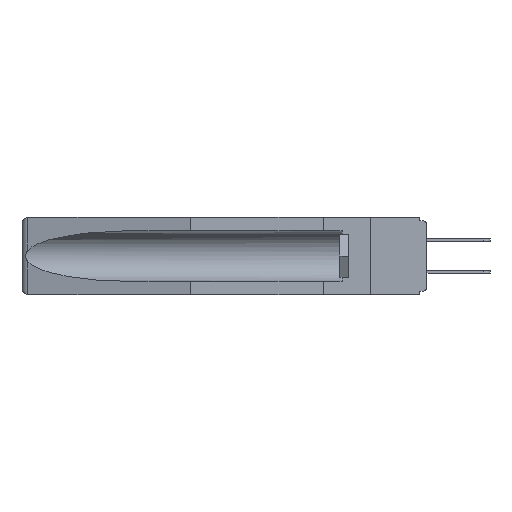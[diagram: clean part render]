
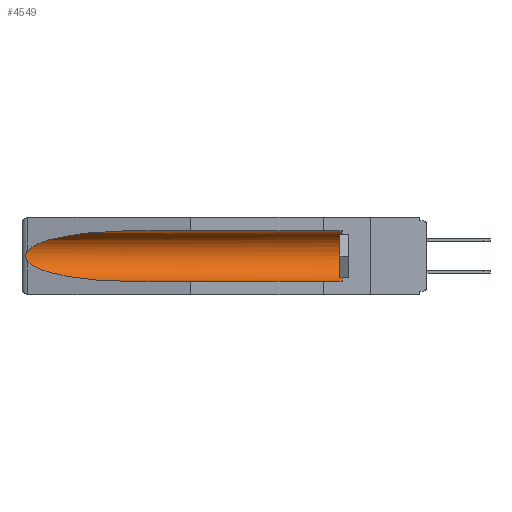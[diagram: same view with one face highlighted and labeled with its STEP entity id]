
A CAD part, left-side view. The second image highlights one B-rep face of the part: STEP entity #4549.
In plain terms, the highlighted cylindrical face has radius 2.857 mm (diameter 5.715 mm), a partial arc.
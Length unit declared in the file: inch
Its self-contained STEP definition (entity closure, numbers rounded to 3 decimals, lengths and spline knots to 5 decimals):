
#113 = DIRECTION ( 'NONE',  ( 0., 1., 0. ) ) ;
#504 = DIRECTION ( 'NONE',  ( 0., 1., 0. ) ) ;
#1116 = CARTESIAN_POINT ( 'NONE',  ( 0.2675, 1.53308, -0.16763 ) ) ;
#1259 = VERTEX_POINT ( 'NONE', #19454 ) ;
#2193 =( BOUNDED_CURVE ( )  B_SPLINE_CURVE ( 3, ( #4883, #7113, #13769, #10383 ),
 .UNSPECIFIED., .F., .F. ) 
 B_SPLINE_CURVE_WITH_KNOTS ( ( 4, 4 ),
 ( 4.71239, 6.08839 ),
 .UNSPECIFIED. ) 
 CURVE ( )  GEOMETRIC_REPRESENTATION_ITEM ( )  RATIONAL_B_SPLINE_CURVE ( ( 1., 0.848, 0.848, 1. ) ) 
 REPRESENTATION_ITEM ( '' )  );
#2358 = CARTESIAN_POINT ( 'NONE',  ( 0.155, 0.126, -0.1715 ) ) ;
#2720 = ORIENTED_EDGE ( 'NONE', *, *, #8087, .T. ) ;
#2957 = CARTESIAN_POINT ( 'NONE',  ( 0.26537, 1.52718, -0.19328 ) ) ;
#4128 = ORIENTED_EDGE ( 'NONE', *, *, #14381, .T. ) ;
#4549 = ADVANCED_FACE ( 'NONE', ( #16466 ), #17534, .F. ) ;
#4883 = CARTESIAN_POINT ( 'NONE',  ( 0.155, 1.07973, -0.059 ) ) ;
#5610 = CARTESIAN_POINT ( 'NONE',  ( 0.26537, 1.52718, -0.19328 ) ) ;
#5616 = CARTESIAN_POINT ( 'NONE',  ( 0.155, 1.07973, -0.059 ) ) ;
#6400 = ORIENTED_EDGE ( 'NONE', *, *, #9458, .T. ) ;
#6553 = EDGE_CURVE ( 'NONE', #7115, #1259, #11115, .T. ) ;
#7113 = CARTESIAN_POINT ( 'NONE',  ( 0.21114, 1.30732, -0.059 ) ) ;
#7115 = VERTEX_POINT ( 'NONE', #13601 ) ;
#7125 = ORIENTED_EDGE ( 'NONE', *, *, #8230, .T. ) ;
#7286 = CARTESIAN_POINT ( 'NONE',  ( 0.155, -0.30754, -0.059 ) ) ;
#7915 = CARTESIAN_POINT ( 'NONE',  ( 0.26654, 1.53092, -0.15636 ) ) ;
#8087 = EDGE_CURVE ( 'NONE', #13979, #14683, #2193, .T. ) ;
#8230 = EDGE_CURVE ( 'NONE', #7115, #16706, #13160, .T. ) ;
#9458 = EDGE_CURVE ( 'NONE', #14683, #10477, #12387, .T. ) ;
#9552 = CARTESIAN_POINT ( 'NONE',  ( 0.26597, 1.5296, -0.19026 ) ) ;
#9699 = CARTESIAN_POINT ( 'NONE',  ( 0.26655, 1.53094, -0.18657 ) ) ;
#10066 = CARTESIAN_POINT ( 'NONE',  ( 0.25451, 1.48313, -0.24835 ) ) ;
#10142 = CARTESIAN_POINT ( 'NONE',  ( 0.155, 1.07973, -0.284 ) ) ;
#10383 = CARTESIAN_POINT ( 'NONE',  ( 0.26537, 1.52718, -0.14972 ) ) ;
#10477 = VERTEX_POINT ( 'NONE', #5610 ) ;
#10748 = DIRECTION ( 'NONE',  ( 0., -1., 0. ) ) ;
#11115 = LINE ( 'NONE', #20878, #17422 ) ;
#11142 = CARTESIAN_POINT ( 'NONE',  ( 0.155, -0.30754, -0.1715 ) ) ;
#11577 = CARTESIAN_POINT ( 'NONE',  ( 0.2675, 1.53308, -0.17534 ) ) ;
#11649 = ORIENTED_EDGE ( 'NONE', *, *, #6553, .F. ) ;
#12387 = B_SPLINE_CURVE_WITH_KNOTS ( 'NONE', 3,
 ( #21725, #19939, #7915, #16424, #1116, #11577, #18129, #9699, #9552, #2957 ),
 .UNSPECIFIED., .F., .F.,
 ( 4, 2, 2, 2, 4 ),
 ( 0., 0.00029, 0.00058, 0.00087, 0.00117 ),
 .UNSPECIFIED. ) ;
#12775 =( BOUNDED_CURVE ( )  B_SPLINE_CURVE ( 3, ( #20241, #10066, #21948, #10142 ),
 .UNSPECIFIED., .F., .F. ) 
 B_SPLINE_CURVE_WITH_KNOTS ( ( 4, 4 ),
 ( 0.1948, 1.5708 ),
 .UNSPECIFIED. ) 
 CURVE ( )  GEOMETRIC_REPRESENTATION_ITEM ( )  RATIONAL_B_SPLINE_CURVE ( ( 1., 0.848, 0.848, 1. ) ) 
 REPRESENTATION_ITEM ( '' )  );
#13160 = CIRCLE ( 'NONE', #15058, 0.1125 ) ;
#13601 = CARTESIAN_POINT ( 'NONE',  ( 0.155, 0.126, -0.284 ) ) ;
#13769 = CARTESIAN_POINT ( 'NONE',  ( 0.25451, 1.48313, -0.09465 ) ) ;
#13979 = VERTEX_POINT ( 'NONE', #5616 ) ;
#14013 = LINE ( 'NONE', #7286, #15593 ) ;
#14131 = AXIS2_PLACEMENT_3D ( 'NONE', #11142, #113, #16196 ) ;
#14381 = EDGE_CURVE ( 'NONE', #16706, #13979, #14013, .T. ) ;
#14683 = VERTEX_POINT ( 'NONE', #18893 ) ;
#15058 = AXIS2_PLACEMENT_3D ( 'NONE', #2358, #10748, #17598 ) ;
#15593 = VECTOR ( 'NONE', #504, 39.37008 ) ;
#16196 = DIRECTION ( 'NONE',  ( 0., 0., 1. ) ) ;
#16424 = CARTESIAN_POINT ( 'NONE',  ( 0.2673, 1.5327, -0.16383 ) ) ;
#16466 = FACE_OUTER_BOUND ( 'NONE', #20711, .T. ) ;
#16706 = VERTEX_POINT ( 'NONE', #17997 ) ;
#17422 = VECTOR ( 'NONE', #17571, 39.37008 ) ;
#17534 = CYLINDRICAL_SURFACE ( 'NONE', #14131, 0.1125 ) ;
#17571 = DIRECTION ( 'NONE',  ( 0., 1., 0. ) ) ;
#17598 = DIRECTION ( 'NONE',  ( 0., 0., 1. ) ) ;
#17997 = CARTESIAN_POINT ( 'NONE',  ( 0.155, 0.126, -0.059 ) ) ;
#18129 = CARTESIAN_POINT ( 'NONE',  ( 0.2673, 1.53269, -0.17917 ) ) ;
#18644 = EDGE_CURVE ( 'NONE', #10477, #1259, #12775, .T. ) ;
#18893 = CARTESIAN_POINT ( 'NONE',  ( 0.26537, 1.52718, -0.14972 ) ) ;
#19454 = CARTESIAN_POINT ( 'NONE',  ( 0.155, 1.07973, -0.284 ) ) ;
#19644 = ORIENTED_EDGE ( 'NONE', *, *, #18644, .T. ) ;
#19939 = CARTESIAN_POINT ( 'NONE',  ( 0.26597, 1.52961, -0.15275 ) ) ;
#20241 = CARTESIAN_POINT ( 'NONE',  ( 0.26537, 1.52718, -0.19328 ) ) ;
#20711 = EDGE_LOOP ( 'NONE', ( #2720, #6400, #19644, #11649, #7125, #4128 ) ) ;
#20878 = CARTESIAN_POINT ( 'NONE',  ( 0.155, -0.30754, -0.284 ) ) ;
#21725 = CARTESIAN_POINT ( 'NONE',  ( 0.26537, 1.52718, -0.14972 ) ) ;
#21948 = CARTESIAN_POINT ( 'NONE',  ( 0.21114, 1.30732, -0.284 ) ) ;
